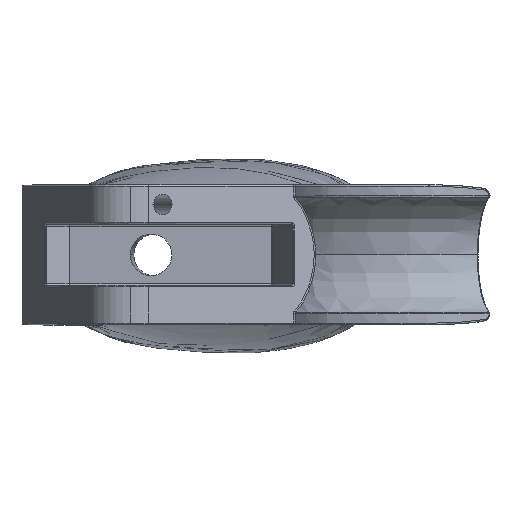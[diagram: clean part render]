
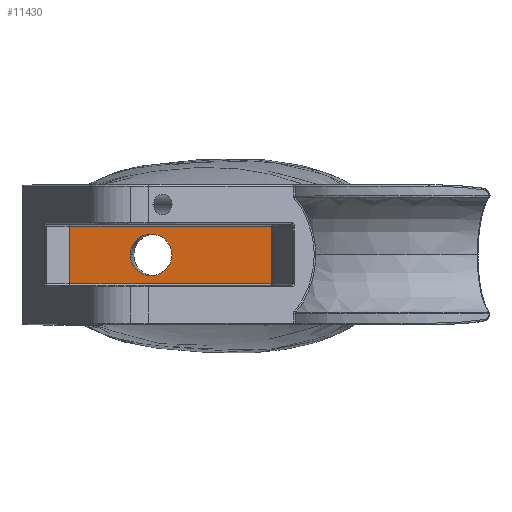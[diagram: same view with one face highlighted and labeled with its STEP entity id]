
A CAD part, top view. The second image highlights one B-rep face of the part: STEP entity #11430.
In plain terms, the highlighted planar face has unit normal (-0.087, 0, 0.996).
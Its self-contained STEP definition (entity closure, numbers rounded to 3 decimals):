
#32 = ORIENTED_EDGE ( 'NONE', *, *, #51171, .F. ) ;
#2214 = VECTOR ( 'NONE', #16543, 1000. ) ;
#5326 = LINE ( 'NONE', #38980, #13521 ) ;
#5760 = ORIENTED_EDGE ( 'NONE', *, *, #36624, .F. ) ;
#6783 = LINE ( 'NONE', #24377, #51595 ) ;
#7206 = VECTOR ( 'NONE', #10865, 1000. ) ;
#8295 = EDGE_CURVE ( 'NONE', #34306, #38334, #6783, .T. ) ;
#8314 = VERTEX_POINT ( 'NONE', #8842 ) ;
#8483 = LINE ( 'NONE', #26387, #7206 ) ;
#8842 = CARTESIAN_POINT ( 'NONE',  ( -7.928, 35.225, 34.027 ) ) ;
#10865 = DIRECTION ( 'NONE',  ( 0., -1., 0. ) ) ;
#11430 = ADVANCED_FACE ( 'NONE', ( #21049, #48220 ), #46617, .F. ) ;
#12408 = DIRECTION ( 'NONE',  ( 0.996, 0., 0.087 ) ) ;
#12757 = ORIENTED_EDGE ( 'NONE', *, *, #8295, .F. ) ;
#12934 = LINE ( 'NONE', #20237, #2214 ) ;
#13521 = VECTOR ( 'NONE', #34870, 1000. ) ;
#13723 = AXIS2_PLACEMENT_3D ( 'NONE', #43461, #31746, #51538 ) ;
#14815 = CARTESIAN_POINT ( 'NONE',  ( -11.167, 35.225, 33.743 ) ) ;
#14972 = EDGE_LOOP ( 'NONE', ( #5760, #12757, #32, #28555 ) ) ;
#15768 = AXIS2_PLACEMENT_3D ( 'NONE', #26450, #46269, #30336 ) ;
#16543 = DIRECTION ( 'NONE',  ( -0.996, 0., -0.087 ) ) ;
#18466 = CARTESIAN_POINT ( 'NONE',  ( 7.601, 30.716, 35.385 ) ) ;
#18469 = EDGE_LOOP ( 'NONE', ( #34262, #26950 ) ) ;
#20237 = CARTESIAN_POINT ( 'NONE',  ( 7.747, 30.716, 35.398 ) ) ;
#21049 = FACE_OUTER_BOUND ( 'NONE', #14972, .T. ) ;
#21952 = CARTESIAN_POINT ( 'NONE',  ( -23.819, 39.733, 32.636 ) ) ;
#22064 = VERTEX_POINT ( 'NONE', #46444 ) ;
#24377 = CARTESIAN_POINT ( 'NONE',  ( 7.747, 39.733, 35.398 ) ) ;
#26387 = CARTESIAN_POINT ( 'NONE',  ( 7.601, 500034.725, 35.385 ) ) ;
#26450 = CARTESIAN_POINT ( 'NONE',  ( 7.747, 500034.725, 35.398 ) ) ;
#26950 = ORIENTED_EDGE ( 'NONE', *, *, #44104, .T. ) ;
#28555 = ORIENTED_EDGE ( 'NONE', *, *, #43101, .F. ) ;
#30336 = DIRECTION ( 'NONE',  ( -0.996, 0., -0.087 ) ) ;
#31746 = DIRECTION ( 'NONE',  ( 0.087, 0., -0.996 ) ) ;
#34262 = ORIENTED_EDGE ( 'NONE', *, *, #49257, .T. ) ;
#34306 = VERTEX_POINT ( 'NONE', #21952 ) ;
#34449 = VERTEX_POINT ( 'NONE', #38931 ) ;
#34870 = DIRECTION ( 'NONE',  ( 0., 1., 0. ) ) ;
#36185 = VERTEX_POINT ( 'NONE', #18466 ) ;
#36624 = EDGE_CURVE ( 'NONE', #38334, #36185, #8483, .T. ) ;
#38334 = VERTEX_POINT ( 'NONE', #51174 ) ;
#38931 = CARTESIAN_POINT ( 'NONE',  ( -23.819, 30.716, 32.636 ) ) ;
#38980 = CARTESIAN_POINT ( 'NONE',  ( -23.819, 500034.725, 32.636 ) ) ;
#39365 = DIRECTION ( 'NONE',  ( 0.996, 0., 0.087 ) ) ;
#39464 = CIRCLE ( 'NONE', #41487, 3.251 ) ;
#39728 = DIRECTION ( 'NONE',  ( 0.087, 0., -0.996 ) ) ;
#41487 = AXIS2_PLACEMENT_3D ( 'NONE', #14815, #39728, #39365 ) ;
#43101 = EDGE_CURVE ( 'NONE', #36185, #34449, #12934, .T. ) ;
#43461 = CARTESIAN_POINT ( 'NONE',  ( -11.167, 35.225, 33.743 ) ) ;
#44104 = EDGE_CURVE ( 'NONE', #22064, #8314, #46843, .T. ) ;
#46269 = DIRECTION ( 'NONE',  ( 0.087, 0., -0.996 ) ) ;
#46444 = CARTESIAN_POINT ( 'NONE',  ( -14.406, 35.225, 33.46 ) ) ;
#46617 = PLANE ( 'NONE',  #15768 ) ;
#46843 = CIRCLE ( 'NONE', #13723, 3.251 ) ;
#48220 = FACE_BOUND ( 'NONE', #18469, .T. ) ;
#49257 = EDGE_CURVE ( 'NONE', #8314, #22064, #39464, .T. ) ;
#51171 = EDGE_CURVE ( 'NONE', #34449, #34306, #5326, .T. ) ;
#51174 = CARTESIAN_POINT ( 'NONE',  ( 7.601, 39.733, 35.385 ) ) ;
#51538 = DIRECTION ( 'NONE',  ( 0.996, 0., 0.087 ) ) ;
#51595 = VECTOR ( 'NONE', #12408, 1000. ) ;
